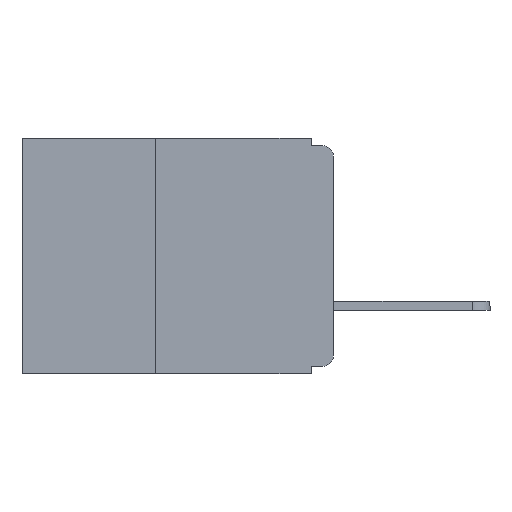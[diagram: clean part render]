
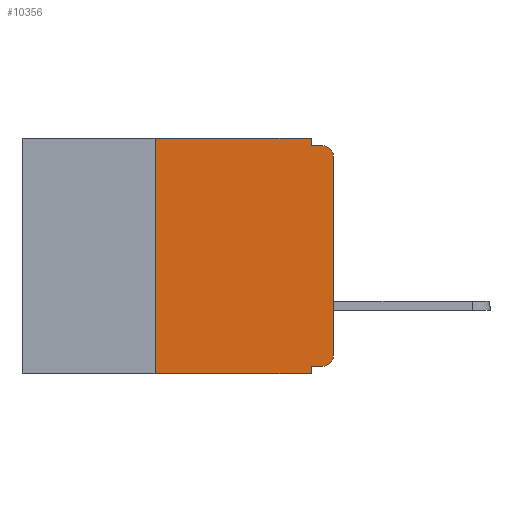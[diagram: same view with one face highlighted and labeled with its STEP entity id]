
A CAD part, left-side view. The second image highlights one B-rep face of the part: STEP entity #10356.
In plain terms, the highlighted planar face has unit normal (-1, 0, 0).
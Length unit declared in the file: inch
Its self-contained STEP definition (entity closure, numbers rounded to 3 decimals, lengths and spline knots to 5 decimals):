
#111 = DIRECTION ( 'NONE',  ( 0., -1., 0. ) ) ;
#187 = CARTESIAN_POINT ( 'NONE',  ( 0., 0., -0.01 ) ) ;
#643 = CARTESIAN_POINT ( 'NONE',  ( 0., 0.031, 0. ) ) ;
#661 = DIRECTION ( 'NONE',  ( 0., 0., -1. ) ) ;
#790 = VECTOR ( 'NONE', #111, 39.37008 ) ;
#825 = LINE ( 'NONE', #187, #790 ) ;
#971 = CARTESIAN_POINT ( 'NONE',  ( 0., 0.031, -0.32 ) ) ;
#1240 = CARTESIAN_POINT ( 'NONE',  ( 0., 0., -0.025 ) ) ;
#1977 = DIRECTION ( 'NONE',  ( 0., -1., 0. ) ) ;
#2256 = VERTEX_POINT ( 'NONE', #4685 ) ;
#2379 = EDGE_CURVE ( 'NONE', #2256, #9214, #5523, .T. ) ;
#2396 = CARTESIAN_POINT ( 'NONE',  ( 0., 0.031, 0. ) ) ;
#2530 = CARTESIAN_POINT ( 'NONE',  ( 0., 0.031, -0.01 ) ) ;
#2587 = CARTESIAN_POINT ( 'NONE',  ( 0., 0.015, -0.01 ) ) ;
#2588 = VERTEX_POINT ( 'NONE', #2530 ) ;
#3250 = VECTOR ( 'NONE', #1977, 39.37008 ) ;
#3512 = CARTESIAN_POINT ( 'NONE',  ( 0., 0.437, -0.33 ) ) ;
#3566 = LINE ( 'NONE', #3512, #3250 ) ;
#4014 = CIRCLE ( 'NONE', #15374, 0.015 ) ;
#4297 = DIRECTION ( 'NONE',  ( 0., 0., -1. ) ) ;
#4301 = DIRECTION ( 'NONE',  ( -1., 0., 0. ) ) ;
#4322 = CARTESIAN_POINT ( 'NONE',  ( 0., 0.015, -0.025 ) ) ;
#4324 = VERTEX_POINT ( 'NONE', #5272 ) ;
#4406 = VERTEX_POINT ( 'NONE', #2396 ) ;
#4581 = EDGE_CURVE ( 'NONE', #2256, #8263, #3566, .T. ) ;
#4685 = CARTESIAN_POINT ( 'NONE',  ( 0., 0.25, -0.33 ) ) ;
#5272 = CARTESIAN_POINT ( 'NONE',  ( 0., 0.015, -0.32 ) ) ;
#5320 = VECTOR ( 'NONE', #12417, 39.37008 ) ;
#5470 = VERTEX_POINT ( 'NONE', #971 ) ;
#5523 = LINE ( 'NONE', #11277, #5320 ) ;
#5587 = VERTEX_POINT ( 'NONE', #13671 ) ;
#5658 = EDGE_CURVE ( 'NONE', #5470, #8263, #15518, .T. ) ;
#5838 = DIRECTION ( 'NONE',  ( 0., 1., 0. ) ) ;
#6040 = CARTESIAN_POINT ( 'NONE',  ( 0., 0., -0.32 ) ) ;
#6907 = CARTESIAN_POINT ( 'NONE',  ( 0., 0., 0. ) ) ;
#6997 = DIRECTION ( 'NONE',  ( 0., 0., 1. ) ) ;
#7114 = ORIENTED_EDGE ( 'NONE', *, *, #12017, .T. ) ;
#7196 = ORIENTED_EDGE ( 'NONE', *, *, #15733, .T. ) ;
#7303 = ORIENTED_EDGE ( 'NONE', *, *, #17479, .F. ) ;
#7635 = ORIENTED_EDGE ( 'NONE', *, *, #16140, .F. ) ;
#7711 = EDGE_CURVE ( 'NONE', #4324, #5470, #12053, .T. ) ;
#7826 = ORIENTED_EDGE ( 'NONE', *, *, #15027, .F. ) ;
#7963 = ORIENTED_EDGE ( 'NONE', *, *, #2379, .F. ) ;
#8075 = ORIENTED_EDGE ( 'NONE', *, *, #4581, .T. ) ;
#8125 = ORIENTED_EDGE ( 'NONE', *, *, #5658, .F. ) ;
#8142 = ORIENTED_EDGE ( 'NONE', *, *, #7711, .F. ) ;
#8263 = VERTEX_POINT ( 'NONE', #14759 ) ;
#8371 = ORIENTED_EDGE ( 'NONE', *, *, #9432, .T. ) ;
#8482 = CARTESIAN_POINT ( 'NONE',  ( 0., 0.031, -0.33 ) ) ;
#8712 = VERTEX_POINT ( 'NONE', #2587 ) ;
#8999 = DIRECTION ( 'NONE',  ( 0., 0., -1. ) ) ;
#9214 = VERTEX_POINT ( 'NONE', #16263 ) ;
#9300 = VECTOR ( 'NONE', #6997, 39.37008 ) ;
#9423 = LINE ( 'NONE', #6907, #9300 ) ;
#9432 = EDGE_CURVE ( 'NONE', #4324, #5587, #4014, .T. ) ;
#9988 = VECTOR ( 'NONE', #661, 39.37008 ) ;
#10104 = LINE ( 'NONE', #643, #9988 ) ;
#10356 = ADVANCED_FACE ( 'NONE', ( #16499 ), #15552, .F. ) ;
#11006 = DIRECTION ( 'NONE',  ( 0., 0., -1. ) ) ;
#11064 = DIRECTION ( 'NONE',  ( -1., 0., 0. ) ) ;
#11066 = CARTESIAN_POINT ( 'NONE',  ( 0., 0.015, -0.305 ) ) ;
#11277 = CARTESIAN_POINT ( 'NONE',  ( 0., 0.25, -0.33 ) ) ;
#11613 = CIRCLE ( 'NONE', #14427, 0.015 ) ;
#11997 = VECTOR ( 'NONE', #5838, 39.37008 ) ;
#12017 = EDGE_CURVE ( 'NONE', #5587, #12595, #9423, .T. ) ;
#12053 = LINE ( 'NONE', #6040, #11997 ) ;
#12417 = DIRECTION ( 'NONE',  ( 0., 0., 1. ) ) ;
#12595 = VERTEX_POINT ( 'NONE', #1240 ) ;
#12970 = CARTESIAN_POINT ( 'NONE',  ( 0., 0.437, 0. ) ) ;
#13084 = DIRECTION ( 'NONE',  ( 0., -1., 0. ) ) ;
#13671 = CARTESIAN_POINT ( 'NONE',  ( 0., 0., -0.305 ) ) ;
#13835 = DIRECTION ( 'NONE',  ( 1., 0., 0. ) ) ;
#14427 = AXIS2_PLACEMENT_3D ( 'NONE', #4322, #4301, #4297 ) ;
#14684 = DIRECTION ( 'NONE',  ( 0., 0., -1. ) ) ;
#14759 = CARTESIAN_POINT ( 'NONE',  ( 0., 0.031, -0.33 ) ) ;
#14889 = CARTESIAN_POINT ( 'NONE',  ( 0., 0.437, 0. ) ) ;
#15027 = EDGE_CURVE ( 'NONE', #9214, #4406, #15287, .T. ) ;
#15126 = VECTOR ( 'NONE', #13084, 39.37008 ) ;
#15287 = LINE ( 'NONE', #12970, #15126 ) ;
#15374 = AXIS2_PLACEMENT_3D ( 'NONE', #11066, #11064, #11006 ) ;
#15383 = VECTOR ( 'NONE', #8999, 39.37008 ) ;
#15518 = LINE ( 'NONE', #8482, #15383 ) ;
#15527 = EDGE_LOOP ( 'NONE', ( #7114, #7196, #7303, #7635, #7826, #7963, #8075, #8125, #8142, #8371 ) ) ;
#15552 = PLANE ( 'NONE',  #16629 ) ;
#15733 = EDGE_CURVE ( 'NONE', #12595, #8712, #11613, .T. ) ;
#16140 = EDGE_CURVE ( 'NONE', #4406, #2588, #10104, .T. ) ;
#16263 = CARTESIAN_POINT ( 'NONE',  ( 0., 0.25, 0. ) ) ;
#16499 = FACE_OUTER_BOUND ( 'NONE', #15527, .T. ) ;
#16629 = AXIS2_PLACEMENT_3D ( 'NONE', #14889, #13835, #14684 ) ;
#17479 = EDGE_CURVE ( 'NONE', #2588, #8712, #825, .T. ) ;
